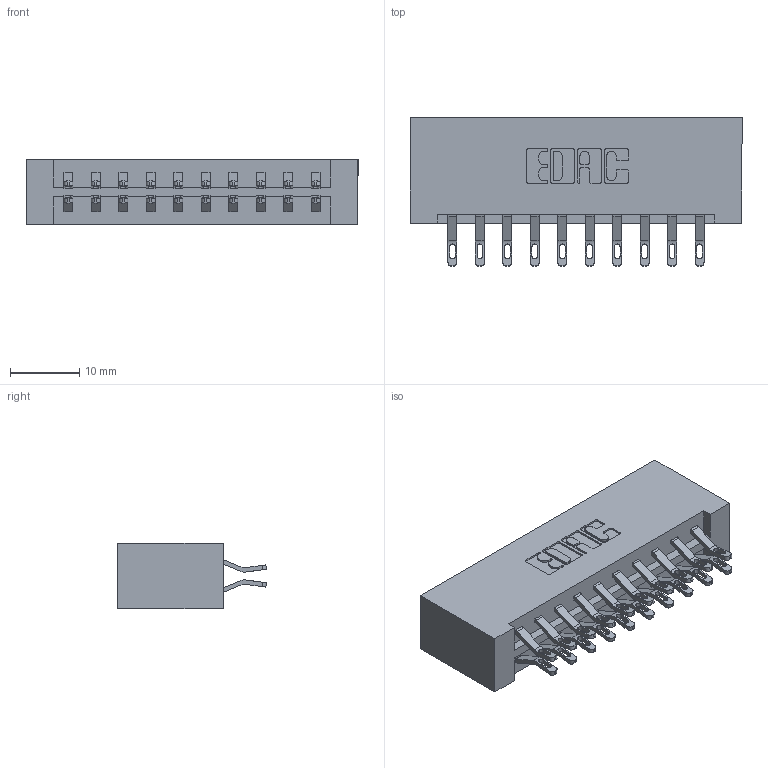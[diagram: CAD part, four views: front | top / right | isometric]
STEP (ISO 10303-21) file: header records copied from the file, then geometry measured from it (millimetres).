
FILE_DESCRIPTION (( 'STEP AP203' ), '1' );
FILE_NAME ('333-020-555-201.STEP', '2018-08-02T00:25:09', ( '' ), ( '' ), 'SwSTEP 2.0', 'SolidWorks 2016', '' );
FILE_SCHEMA (( 'CONFIG_CONTROL_DESIGN' ));
Length unit declared in the file: inch
Products named in the file (3): 333-020-555-201; 333 Part_Lugless; 345-292-001_555 Tail
Assembly tree (21 placements, depth 2):
  333-020-555-201
    333 Part_Lugless
    345-292-001_555 Tail  x20
Bounding box: 47.88 x 21.47 x 9.4 mm (x, y, z)
Volume: 5279.2 mm3; surface area: 6138.7 mm2
Topology: 21 solids, 21 shells, 1266 faces, 3947 edges, 2630 vertices
Faces by surface type: plane 746, cylinder 520
Entity records: 10621 total; most frequent: CARTESIAN_POINT 1832, ORIENTED_EDGE 1738, DIRECTION 1585, EDGE_CURVE 869, LINE 729, VECTOR 729, VERTEX_POINT 578, AXIS2_PLACEMENT_3D 428
